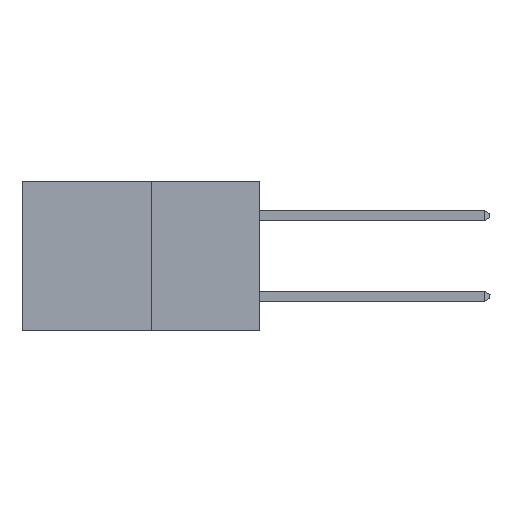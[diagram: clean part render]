
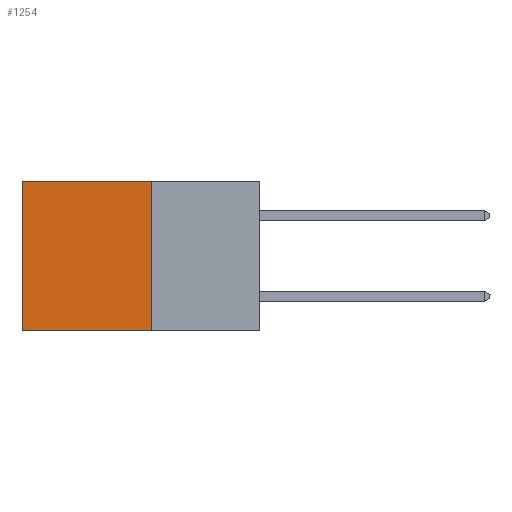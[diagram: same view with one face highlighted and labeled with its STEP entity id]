
A CAD part, left-side view. The second image highlights one B-rep face of the part: STEP entity #1254.
In plain terms, the highlighted planar face has unit normal (-1, 0, 0).
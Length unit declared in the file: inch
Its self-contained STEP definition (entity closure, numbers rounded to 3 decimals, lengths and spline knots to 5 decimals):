
#12 = ORIENTED_EDGE ( 'NONE', *, *, #1713, .T. ) ;
#148 = DIRECTION ( 'NONE',  ( 0., 1., 0. ) ) ;
#301 = CARTESIAN_POINT ( 'NONE',  ( 0.277, 0.27, 0. ) ) ;
#609 = ORIENTED_EDGE ( 'NONE', *, *, #4364, .F. ) ;
#1087 = CARTESIAN_POINT ( 'NONE',  ( 0.277, 0.27, -0.37 ) ) ;
#1240 = CARTESIAN_POINT ( 'NONE',  ( 0.277, 0.27, -0.37 ) ) ;
#1254 = ADVANCED_FACE ( 'NONE', ( #8841 ), #8234, .F. ) ;
#1587 = ORIENTED_EDGE ( 'NONE', *, *, #1978, .T. ) ;
#1713 = EDGE_CURVE ( 'NONE', #5194, #5549, #4250, .T. ) ;
#1741 = VECTOR ( 'NONE', #148, 39.37008 ) ;
#1978 = EDGE_CURVE ( 'NONE', #5549, #4261, #4820, .T. ) ;
#2867 = ORIENTED_EDGE ( 'NONE', *, *, #4722, .F. ) ;
#3123 = CARTESIAN_POINT ( 'NONE',  ( 0.277, 0.59, -0.37 ) ) ;
#3733 = CARTESIAN_POINT ( 'NONE',  ( 0.277, 0.27, -0.37 ) ) ;
#3815 = LINE ( 'NONE', #5192, #7367 ) ;
#4179 = DIRECTION ( 'NONE',  ( 1., 0., 0. ) ) ;
#4250 = LINE ( 'NONE', #301, #1741 ) ;
#4261 = VERTEX_POINT ( 'NONE', #3123 ) ;
#4364 = EDGE_CURVE ( 'NONE', #6531, #4261, #6654, .T. ) ;
#4573 = VECTOR ( 'NONE', #5378, 39.37008 ) ;
#4722 = EDGE_CURVE ( 'NONE', #5194, #6531, #3815, .T. ) ;
#4820 = LINE ( 'NONE', #8551, #6412 ) ;
#4971 = CARTESIAN_POINT ( 'NONE',  ( 0.277, 0.27, 0. ) ) ;
#5192 = CARTESIAN_POINT ( 'NONE',  ( 0.277, 0.27, -0.37 ) ) ;
#5194 = VERTEX_POINT ( 'NONE', #4971 ) ;
#5316 = CARTESIAN_POINT ( 'NONE',  ( 0.277, 0.59, 0. ) ) ;
#5378 = DIRECTION ( 'NONE',  ( 0., 1., 0. ) ) ;
#5549 = VERTEX_POINT ( 'NONE', #5316 ) ;
#6301 = EDGE_LOOP ( 'NONE', ( #1587, #609, #2867, #12 ) ) ;
#6358 = DIRECTION ( 'NONE',  ( 0., 0., -1. ) ) ;
#6412 = VECTOR ( 'NONE', #6608, 39.37008 ) ;
#6531 = VERTEX_POINT ( 'NONE', #1240 ) ;
#6608 = DIRECTION ( 'NONE',  ( 0., 0., -1. ) ) ;
#6654 = LINE ( 'NONE', #3733, #4573 ) ;
#7195 = AXIS2_PLACEMENT_3D ( 'NONE', #1087, #4179, #6358 ) ;
#7367 = VECTOR ( 'NONE', #8785, 39.37008 ) ;
#8234 = PLANE ( 'NONE',  #7195 ) ;
#8551 = CARTESIAN_POINT ( 'NONE',  ( 0.277, 0.59, -0.37 ) ) ;
#8785 = DIRECTION ( 'NONE',  ( 0., 0., -1. ) ) ;
#8841 = FACE_OUTER_BOUND ( 'NONE', #6301, .T. ) ;
